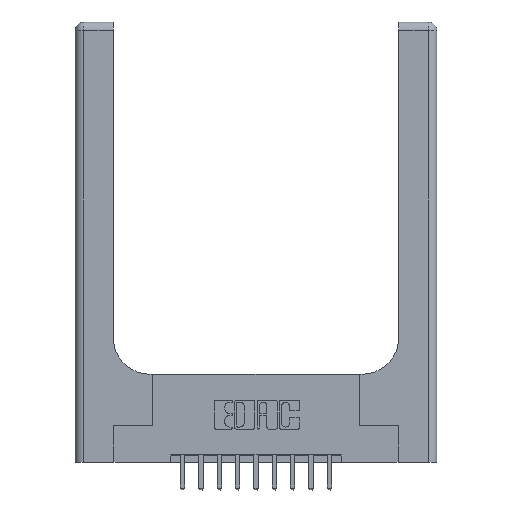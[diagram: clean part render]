
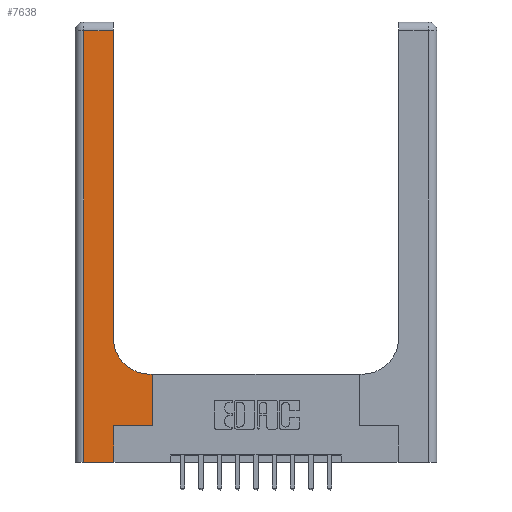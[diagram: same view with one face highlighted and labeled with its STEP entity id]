
A CAD part, top view. The second image highlights one B-rep face of the part: STEP entity #7638.
In plain terms, the highlighted planar face has unit normal (0, 0, 1).
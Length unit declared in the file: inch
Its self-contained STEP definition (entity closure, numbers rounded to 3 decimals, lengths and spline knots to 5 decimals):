
#109 = CARTESIAN_POINT ( 'NONE',  ( 0.265, 0.25, 0.37 ) ) ;
#135 = VERTEX_POINT ( 'NONE', #6908 ) ;
#217 = LINE ( 'NONE', #10191, #15207 ) ;
#376 = VERTEX_POINT ( 'NONE', #386 ) ;
#386 = CARTESIAN_POINT ( 'NONE',  ( 0.06, 2.94, 0.37 ) ) ;
#498 = VECTOR ( 'NONE', #1827, 39.37008 ) ;
#627 = DIRECTION ( 'NONE',  ( 0., 0., -1. ) ) ;
#700 = CARTESIAN_POINT ( 'NONE',  ( 0.265, 0.25, 0.37 ) ) ;
#756 = LINE ( 'NONE', #10562, #15754 ) ;
#1007 = VERTEX_POINT ( 'NONE', #9551 ) ;
#1036 = EDGE_CURVE ( 'NONE', #15436, #135, #8315, .T. ) ;
#1477 = DIRECTION ( 'NONE',  ( 0., 0., -1. ) ) ;
#1827 = DIRECTION ( 'NONE',  ( 0., 1., 0. ) ) ;
#1941 = DIRECTION ( 'NONE',  ( -1., 0., 0. ) ) ;
#2197 = CARTESIAN_POINT ( 'NONE',  ( 0., 2.94, 0.37 ) ) ;
#2274 = LINE ( 'NONE', #2197, #9056 ) ;
#2294 = CARTESIAN_POINT ( 'NONE',  ( 0.06, 0., 0.37 ) ) ;
#3053 = ORIENTED_EDGE ( 'NONE', *, *, #14012, .T. ) ;
#3165 = DIRECTION ( 'NONE',  ( -1., 0., 0. ) ) ;
#3315 = DIRECTION ( 'NONE',  ( -1., 0., 0. ) ) ;
#4043 = AXIS2_PLACEMENT_3D ( 'NONE', #4579, #627, #9211 ) ;
#4062 = EDGE_CURVE ( 'NONE', #6295, #1007, #9189, .T. ) ;
#4304 = EDGE_CURVE ( 'NONE', #1007, #376, #2274, .T. ) ;
#4414 = EDGE_CURVE ( 'NONE', #15732, #10623, #8930, .T. ) ;
#4579 = CARTESIAN_POINT ( 'NONE',  ( 0.51, 0.85, 0.37 ) ) ;
#4744 = VERTEX_POINT ( 'NONE', #2294 ) ;
#5048 = ORIENTED_EDGE ( 'NONE', *, *, #1036, .T. ) ;
#5345 = LINE ( 'NONE', #6811, #13653 ) ;
#5478 = ORIENTED_EDGE ( 'NONE', *, *, #4414, .T. ) ;
#6215 = ORIENTED_EDGE ( 'NONE', *, *, #4304, .T. ) ;
#6295 = VERTEX_POINT ( 'NONE', #11601 ) ;
#6560 = DIRECTION ( 'NONE',  ( 1., 0., 0. ) ) ;
#6811 = CARTESIAN_POINT ( 'NONE',  ( 0., 0., 0.37 ) ) ;
#6908 = CARTESIAN_POINT ( 'NONE',  ( 0.51, 0.6, 0.37 ) ) ;
#7072 = EDGE_LOOP ( 'NONE', ( #7828, #6215, #9291, #15209, #3053, #5478, #15693, #5048, #9217 ) ) ;
#7153 = VERTEX_POINT ( 'NONE', #12368 ) ;
#7399 = DIRECTION ( 'NONE',  ( 1., 0., 0. ) ) ;
#7620 = FACE_OUTER_BOUND ( 'NONE', #7072, .T. ) ;
#7638 = ADVANCED_FACE ( 'NONE', ( #7620 ), #12566, .F. ) ;
#7828 = ORIENTED_EDGE ( 'NONE', *, *, #4062, .T. ) ;
#7872 = CARTESIAN_POINT ( 'NONE',  ( 0.528, 0.25, 0.37 ) ) ;
#7974 = CARTESIAN_POINT ( 'NONE',  ( 0.26, 3., 0.37 ) ) ;
#8315 = LINE ( 'NONE', #13291, #9605 ) ;
#8930 = LINE ( 'NONE', #109, #12416 ) ;
#9056 = VECTOR ( 'NONE', #3315, 39.37008 ) ;
#9189 = LINE ( 'NONE', #7974, #498 ) ;
#9211 = DIRECTION ( 'NONE',  ( 1., 0., 0. ) ) ;
#9217 = ORIENTED_EDGE ( 'NONE', *, *, #14204, .T. ) ;
#9291 = ORIENTED_EDGE ( 'NONE', *, *, #14923, .T. ) ;
#9551 = CARTESIAN_POINT ( 'NONE',  ( 0.26, 2.94, 0.37 ) ) ;
#9605 = VECTOR ( 'NONE', #1941, 39.37008 ) ;
#10191 = CARTESIAN_POINT ( 'NONE',  ( 0.265, 0., 0.37 ) ) ;
#10312 = DIRECTION ( 'NONE',  ( 0., -1., 0. ) ) ;
#10420 = CARTESIAN_POINT ( 'NONE',  ( 0.528, 0.25, 0.37 ) ) ;
#10536 = VECTOR ( 'NONE', #12923, 39.37008 ) ;
#10562 = CARTESIAN_POINT ( 'NONE',  ( 0.06, 3., 0.37 ) ) ;
#10623 = VERTEX_POINT ( 'NONE', #7872 ) ;
#11305 = AXIS2_PLACEMENT_3D ( 'NONE', #11362, #1477, #3165 ) ;
#11362 = CARTESIAN_POINT ( 'NONE',  ( 0., 3., 0.37 ) ) ;
#11568 = CIRCLE ( 'NONE', #4043, 0.25 ) ;
#11601 = CARTESIAN_POINT ( 'NONE',  ( 0.26, 0.85, 0.37 ) ) ;
#12120 = CARTESIAN_POINT ( 'NONE',  ( 0.528, 0.6, 0.37 ) ) ;
#12368 = CARTESIAN_POINT ( 'NONE',  ( 0.265, 0., 0.37 ) ) ;
#12416 = VECTOR ( 'NONE', #7399, 39.37008 ) ;
#12566 = PLANE ( 'NONE',  #11305 ) ;
#12841 = LINE ( 'NONE', #10420, #10536 ) ;
#12923 = DIRECTION ( 'NONE',  ( 0., 1., 0. ) ) ;
#13291 = CARTESIAN_POINT ( 'NONE',  ( 0.26, 0.6, 0.37 ) ) ;
#13653 = VECTOR ( 'NONE', #6560, 39.37008 ) ;
#14012 = EDGE_CURVE ( 'NONE', #7153, #15732, #217, .T. ) ;
#14204 = EDGE_CURVE ( 'NONE', #135, #6295, #11568, .T. ) ;
#14579 = EDGE_CURVE ( 'NONE', #10623, #15436, #12841, .T. ) ;
#14906 = EDGE_CURVE ( 'NONE', #4744, #7153, #5345, .T. ) ;
#14923 = EDGE_CURVE ( 'NONE', #376, #4744, #756, .T. ) ;
#15207 = VECTOR ( 'NONE', #15326, 39.37008 ) ;
#15209 = ORIENTED_EDGE ( 'NONE', *, *, #14906, .T. ) ;
#15326 = DIRECTION ( 'NONE',  ( 0., 1., 0. ) ) ;
#15436 = VERTEX_POINT ( 'NONE', #12120 ) ;
#15693 = ORIENTED_EDGE ( 'NONE', *, *, #14579, .T. ) ;
#15732 = VERTEX_POINT ( 'NONE', #700 ) ;
#15754 = VECTOR ( 'NONE', #10312, 39.37008 ) ;
